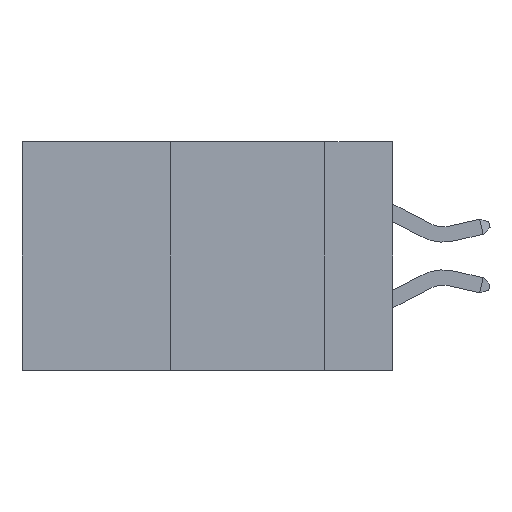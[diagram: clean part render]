
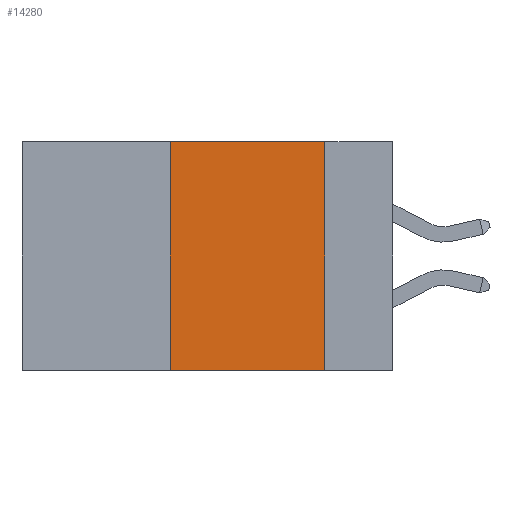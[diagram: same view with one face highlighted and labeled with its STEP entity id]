
A CAD part, left-side view. The second image highlights one B-rep face of the part: STEP entity #14280.
In plain terms, the highlighted planar face has unit normal (-1, 0, 0).
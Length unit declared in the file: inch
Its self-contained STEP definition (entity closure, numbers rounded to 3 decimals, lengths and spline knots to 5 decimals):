
#1428 = ORIENTED_EDGE ( 'NONE', *, *, #14240, .F. ) ;
#2714 = VECTOR ( 'NONE', #5745, 39.37008 ) ;
#3385 = LINE ( 'NONE', #22332, #17833 ) ;
#3544 = DIRECTION ( 'NONE',  ( 0., -1., 0. ) ) ;
#3720 = CARTESIAN_POINT ( 'NONE',  ( 0., 0.6, 0. ) ) ;
#3743 = CARTESIAN_POINT ( 'NONE',  ( 0., 0.6, -0.37 ) ) ;
#4747 = EDGE_CURVE ( 'NONE', #13419, #13972, #3385, .T. ) ;
#4850 = ORIENTED_EDGE ( 'NONE', *, *, #15122, .T. ) ;
#5080 = ORIENTED_EDGE ( 'NONE', *, *, #13872, .F. ) ;
#5745 = DIRECTION ( 'NONE',  ( 0., -1., 0. ) ) ;
#5921 = VERTEX_POINT ( 'NONE', #19370 ) ;
#7725 = FACE_OUTER_BOUND ( 'NONE', #21585, .T. ) ;
#9467 = CARTESIAN_POINT ( 'NONE',  ( 0., 0.36, 0. ) ) ;
#11340 = DIRECTION ( 'NONE',  ( 0., 0., -1. ) ) ;
#11573 = VERTEX_POINT ( 'NONE', #11703 ) ;
#11703 = CARTESIAN_POINT ( 'NONE',  ( 0., 0.36, 0. ) ) ;
#11773 = CARTESIAN_POINT ( 'NONE',  ( 0., 0.11, -0.37 ) ) ;
#11956 = ORIENTED_EDGE ( 'NONE', *, *, #4747, .F. ) ;
#13019 = LINE ( 'NONE', #20615, #16602 ) ;
#13419 = VERTEX_POINT ( 'NONE', #17782 ) ;
#13697 = DIRECTION ( 'NONE',  ( 1., 0., 0. ) ) ;
#13872 = EDGE_CURVE ( 'NONE', #11573, #13419, #13019, .T. ) ;
#13972 = VERTEX_POINT ( 'NONE', #11773 ) ;
#14240 = EDGE_CURVE ( 'NONE', #5921, #11573, #15563, .T. ) ;
#14280 = ADVANCED_FACE ( 'NONE', ( #7725 ), #22791, .F. ) ;
#14742 = DIRECTION ( 'NONE',  ( 0., 0., -1. ) ) ;
#15122 = EDGE_CURVE ( 'NONE', #5921, #13972, #22810, .T. ) ;
#15563 = LINE ( 'NONE', #9467, #23796 ) ;
#16602 = VECTOR ( 'NONE', #3544, 39.37008 ) ;
#17782 = CARTESIAN_POINT ( 'NONE',  ( 0., 0.11, 0. ) ) ;
#17833 = VECTOR ( 'NONE', #14742, 39.37008 ) ;
#19370 = CARTESIAN_POINT ( 'NONE',  ( 0., 0.36, -0.37 ) ) ;
#20615 = CARTESIAN_POINT ( 'NONE',  ( 0., 0.6, 0. ) ) ;
#21050 = DIRECTION ( 'NONE',  ( 0., 0., 1. ) ) ;
#21585 = EDGE_LOOP ( 'NONE', ( #11956, #5080, #1428, #4850 ) ) ;
#22332 = CARTESIAN_POINT ( 'NONE',  ( 0., 0.11, 0. ) ) ;
#22791 = PLANE ( 'NONE',  #24190 ) ;
#22810 = LINE ( 'NONE', #3743, #2714 ) ;
#23796 = VECTOR ( 'NONE', #21050, 39.37008 ) ;
#24190 = AXIS2_PLACEMENT_3D ( 'NONE', #3720, #13697, #11340 ) ;
